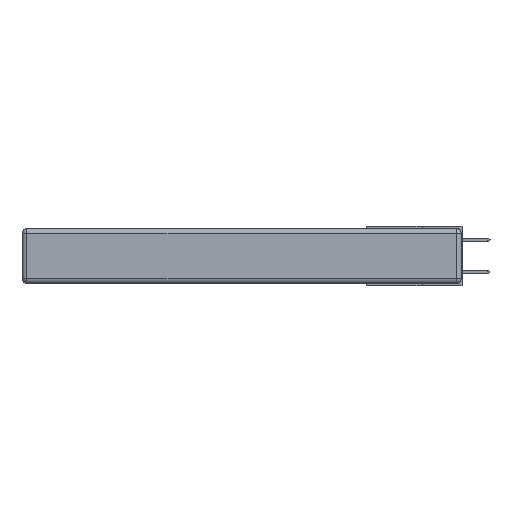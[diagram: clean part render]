
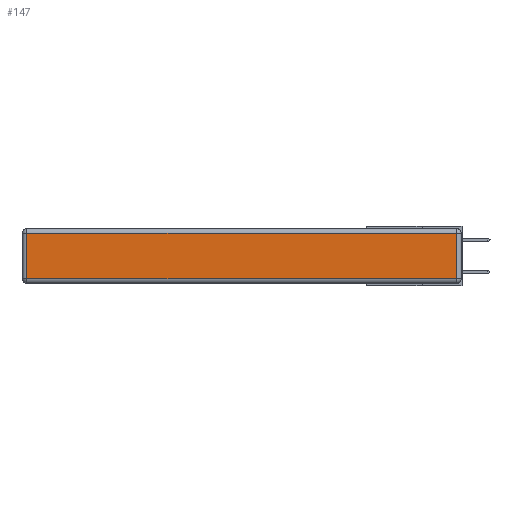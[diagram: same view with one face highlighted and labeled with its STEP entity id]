
A CAD part, left-side view. The second image highlights one B-rep face of the part: STEP entity #147.
In plain terms, the highlighted planar face has unit normal (-1, 0, 0).
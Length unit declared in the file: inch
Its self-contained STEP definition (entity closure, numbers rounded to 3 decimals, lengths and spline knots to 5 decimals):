
#147 = ADVANCED_FACE ( 'NONE', ( #1477 ), #4012, .T. ) ;
#386 = LINE ( 'NONE', #9360, #13379 ) ;
#500 = VERTEX_POINT ( 'NONE', #3074 ) ;
#1198 = EDGE_CURVE ( 'NONE', #14655, #27332, #22598, .T. ) ;
#1477 = FACE_OUTER_BOUND ( 'NONE', #21736, .T. ) ;
#1626 = CARTESIAN_POINT ( 'NONE',  ( 0., 0.03, -0.313 ) ) ;
#3074 = CARTESIAN_POINT ( 'NONE',  ( 0., 2.72, -0.313 ) ) ;
#4012 = PLANE ( 'NONE',  #23980 ) ;
#4208 = ORIENTED_EDGE ( 'NONE', *, *, #28279, .T. ) ;
#4304 = DIRECTION ( 'NONE',  ( 0., 0., 1. ) ) ;
#9360 = CARTESIAN_POINT ( 'NONE',  ( 0., 2.72, -0.343 ) ) ;
#11565 = DIRECTION ( 'NONE',  ( 0., 0., -1. ) ) ;
#12132 = ORIENTED_EDGE ( 'NONE', *, *, #1198, .T. ) ;
#13174 = EDGE_CURVE ( 'NONE', #16550, #500, #386, .T. ) ;
#13379 = VECTOR ( 'NONE', #11565, 39.37008 ) ;
#14112 = CARTESIAN_POINT ( 'NONE',  ( 0., 2.75, -0.03 ) ) ;
#14655 = VERTEX_POINT ( 'NONE', #1626 ) ;
#16222 = DIRECTION ( 'NONE',  ( 0., 1., 0. ) ) ;
#16550 = VERTEX_POINT ( 'NONE', #18228 ) ;
#17314 = DIRECTION ( 'NONE',  ( 0., 0., 1. ) ) ;
#18228 = CARTESIAN_POINT ( 'NONE',  ( 0., 2.72, -0.03 ) ) ;
#18864 = VECTOR ( 'NONE', #24034, 39.37008 ) ;
#19212 = VECTOR ( 'NONE', #16222, 39.37008 ) ;
#19382 = CARTESIAN_POINT ( 'NONE',  ( 0., 0., -0.343 ) ) ;
#19502 = ORIENTED_EDGE ( 'NONE', *, *, #26500, .T. ) ;
#19689 = CARTESIAN_POINT ( 'NONE',  ( 0., 0., -0.313 ) ) ;
#21736 = EDGE_LOOP ( 'NONE', ( #4208, #12132, #19502, #24870 ) ) ;
#22030 = DIRECTION ( 'NONE',  ( -1., 0., 0. ) ) ;
#22598 = LINE ( 'NONE', #25943, #24289 ) ;
#22614 = LINE ( 'NONE', #14112, #19212 ) ;
#22740 = CARTESIAN_POINT ( 'NONE',  ( 0., 0.03, -0.03 ) ) ;
#23980 = AXIS2_PLACEMENT_3D ( 'NONE', #19382, #22030, #4304 ) ;
#24034 = DIRECTION ( 'NONE',  ( 0., -1., 0. ) ) ;
#24289 = VECTOR ( 'NONE', #17314, 39.37008 ) ;
#24870 = ORIENTED_EDGE ( 'NONE', *, *, #13174, .T. ) ;
#25943 = CARTESIAN_POINT ( 'NONE',  ( 0., 0.03, -0.343 ) ) ;
#26244 = LINE ( 'NONE', #19689, #18864 ) ;
#26500 = EDGE_CURVE ( 'NONE', #27332, #16550, #22614, .T. ) ;
#27332 = VERTEX_POINT ( 'NONE', #22740 ) ;
#28279 = EDGE_CURVE ( 'NONE', #500, #14655, #26244, .T. ) ;
